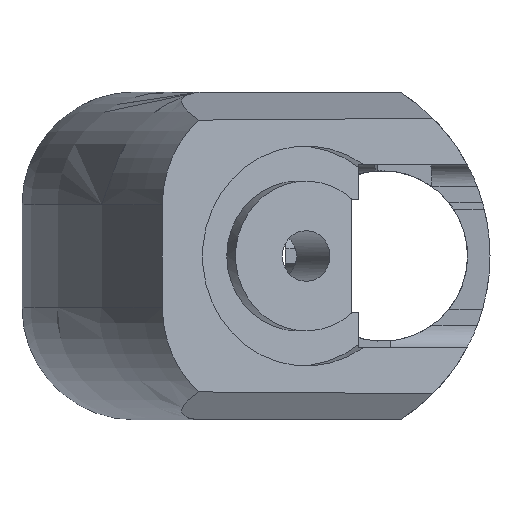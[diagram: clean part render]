
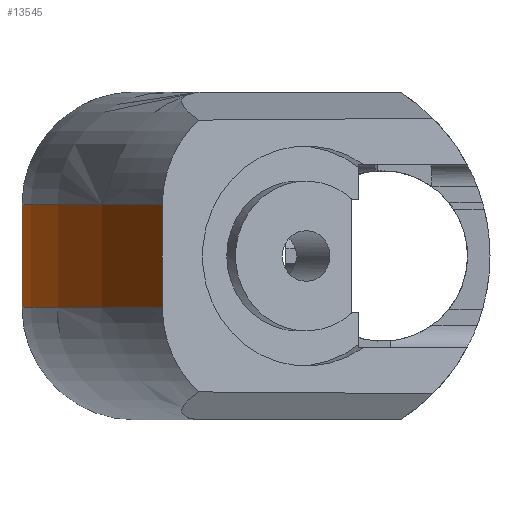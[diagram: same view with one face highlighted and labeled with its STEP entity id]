
A CAD part, left-side view. The second image highlights one B-rep face of the part: STEP entity #13545.
In plain terms, the highlighted cylindrical face has radius 197.297 mm (diameter 394.594 mm), a partial arc.
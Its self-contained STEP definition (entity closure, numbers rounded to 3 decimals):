
#157 = PLANE('',#158);
#158 = AXIS2_PLACEMENT_3D('',#159,#160,#161);
#159 = CARTESIAN_POINT('',(0.,63.5,-22.225));
#160 = DIRECTION('',(0.,-1.,0.));
#161 = DIRECTION('',(-1.,0.,0.));
#2285 = PLANE('',#2286);
#2286 = AXIS2_PLACEMENT_3D('',#2287,#2288,#2289);
#2287 = CARTESIAN_POINT('',(-209.55,44.45,-22.225));
#2288 = DIRECTION('',(0.943,0.334,0.)
  );
#2289 = DIRECTION('',(0.334,-0.943,0.)
  );
#2979 = TOROIDAL_SURFACE('',#2980,182.057,15.24);
#2980 = AXIS2_PLACEMENT_3D('',#2981,#2982,#2983);
#2981 = CARTESIAN_POINT('',(-124.968,-133.797,6.985));
#2982 = DIRECTION('',(0.,0.,-1.));
#2983 = DIRECTION('',(0.,1.,0.));
#4018 = VERTEX_POINT('',#4019);
#4019 = CARTESIAN_POINT('',(-124.968,63.5,6.985));
#4344 = EDGE_CURVE('',#4345,#4018,#4347,.T.);
#4345 = VERTEX_POINT('',#4346);
#4346 = CARTESIAN_POINT('',(-124.968,63.5,-6.985));
#4347 = SURFACE_CURVE('',#4348,(#4352,#4359),.PCURVE_S1.);
#4348 = LINE('',#4349,#4350);
#4349 = CARTESIAN_POINT('',(-124.968,63.5,-22.225));
#4350 = VECTOR('',#4351,1.);
#4351 = DIRECTION('',(0.,0.,1.));
#4352 = PCURVE('',#157,#4353);
#4353 = DEFINITIONAL_REPRESENTATION('',(#4354),#4358);
#4354 = LINE('',#4355,#4356);
#4355 = CARTESIAN_POINT('',(124.968,0.));
#4356 = VECTOR('',#4357,1.);
#4357 = DIRECTION('',(0.,-1.));
#4358 = ( GEOMETRIC_REPRESENTATION_CONTEXT(2) 
PARAMETRIC_REPRESENTATION_CONTEXT() REPRESENTATION_CONTEXT('2D SPACE',''
  ) );
#4359 = PCURVE('',#4360,#4365);
#4360 = CYLINDRICAL_SURFACE('',#4361,197.297);
#4361 = AXIS2_PLACEMENT_3D('',#4362,#4363,#4364);
#4362 = CARTESIAN_POINT('',(-124.968,-133.797,-22.225));
#4363 = DIRECTION('',(0.,0.,-1.));
#4364 = DIRECTION('',(1.,0.,0.));
#4365 = DEFINITIONAL_REPRESENTATION('',(#4366),#4370);
#4366 = LINE('',#4367,#4368);
#4367 = CARTESIAN_POINT('',(-1.571,0.));
#4368 = VECTOR('',#4369,1.);
#4369 = DIRECTION('',(-0.,-1.));
#4370 = ( GEOMETRIC_REPRESENTATION_CONTEXT(2) 
PARAMETRIC_REPRESENTATION_CONTEXT() REPRESENTATION_CONTEXT('2D SPACE',''
  ) );
#4468 = TOROIDAL_SURFACE('',#4469,182.057,15.24);
#4469 = AXIS2_PLACEMENT_3D('',#4470,#4471,#4472);
#4470 = CARTESIAN_POINT('',(-124.968,-133.797,-6.985));
#4471 = DIRECTION('',(0.,0.,1.));
#4472 = DIRECTION('',(0.,1.,0.));
#10113 = VERTEX_POINT('',#10114);
#10114 = CARTESIAN_POINT('',(-209.55,44.45,-6.985));
#10204 = EDGE_CURVE('',#10113,#10205,#10207,.T.);
#10205 = VERTEX_POINT('',#10206);
#10206 = CARTESIAN_POINT('',(-209.55,44.45,6.985));
#10207 = SURFACE_CURVE('',#10208,(#10212,#10219),.PCURVE_S1.);
#10208 = LINE('',#10209,#10210);
#10209 = CARTESIAN_POINT('',(-209.55,44.45,-22.225));
#10210 = VECTOR('',#10211,1.);
#10211 = DIRECTION('',(0.,0.,1.));
#10212 = PCURVE('',#2285,#10213);
#10213 = DEFINITIONAL_REPRESENTATION('',(#10214),#10218);
#10214 = LINE('',#10215,#10216);
#10215 = CARTESIAN_POINT('',(0.,-0.));
#10216 = VECTOR('',#10217,1.);
#10217 = DIRECTION('',(0.,-1.));
#10218 = ( GEOMETRIC_REPRESENTATION_CONTEXT(2) 
PARAMETRIC_REPRESENTATION_CONTEXT() REPRESENTATION_CONTEXT('2D SPACE',''
  ) );
#10219 = PCURVE('',#4360,#10220);
#10220 = DEFINITIONAL_REPRESENTATION('',(#10221),#10225);
#10221 = LINE('',#10222,#10223);
#10222 = CARTESIAN_POINT('',(-2.014,0.));
#10223 = VECTOR('',#10224,1.);
#10224 = DIRECTION('',(-0.,-1.));
#10225 = ( GEOMETRIC_REPRESENTATION_CONTEXT(2) 
PARAMETRIC_REPRESENTATION_CONTEXT() REPRESENTATION_CONTEXT('2D SPACE',''
  ) );
#11246 = EDGE_CURVE('',#4018,#10205,#11247,.T.);
#11247 = SURFACE_CURVE('',#11248,(#11253,#11260),.PCURVE_S1.);
#11248 = CIRCLE('',#11249,197.297);
#11249 = AXIS2_PLACEMENT_3D('',#11250,#11251,#11252);
#11250 = CARTESIAN_POINT('',(-124.968,-133.797,6.985));
#11251 = DIRECTION('',(0.,0.,1.));
#11252 = DIRECTION('',(0.,1.,0.));
#11253 = PCURVE('',#2979,#11254);
#11254 = DEFINITIONAL_REPRESENTATION('',(#11255),#11259);
#11255 = LINE('',#11256,#11257);
#11256 = CARTESIAN_POINT('',(-0.,6.283));
#11257 = VECTOR('',#11258,1.);
#11258 = DIRECTION('',(-1.,0.));
#11259 = ( GEOMETRIC_REPRESENTATION_CONTEXT(2) 
PARAMETRIC_REPRESENTATION_CONTEXT() REPRESENTATION_CONTEXT('2D SPACE',''
  ) );
#11260 = PCURVE('',#4360,#11261);
#11261 = DEFINITIONAL_REPRESENTATION('',(#11262),#11266);
#11262 = LINE('',#11263,#11264);
#11263 = CARTESIAN_POINT('',(-1.571,-29.21));
#11264 = VECTOR('',#11265,1.);
#11265 = DIRECTION('',(-1.,0.));
#11266 = ( GEOMETRIC_REPRESENTATION_CONTEXT(2) 
PARAMETRIC_REPRESENTATION_CONTEXT() REPRESENTATION_CONTEXT('2D SPACE',''
  ) );
#13545 = ADVANCED_FACE('',(#13546),#4360,.T.);
#13546 = FACE_BOUND('',#13547,.F.);
#13547 = EDGE_LOOP('',(#13548,#13549,#13550,#13551));
#13548 = ORIENTED_EDGE('',*,*,#4344,.T.);
#13549 = ORIENTED_EDGE('',*,*,#11246,.T.);
#13550 = ORIENTED_EDGE('',*,*,#10204,.F.);
#13551 = ORIENTED_EDGE('',*,*,#13552,.F.);
#13552 = EDGE_CURVE('',#4345,#10113,#13553,.T.);
#13553 = SURFACE_CURVE('',#13554,(#13559,#13566),.PCURVE_S1.);
#13554 = CIRCLE('',#13555,197.297);
#13555 = AXIS2_PLACEMENT_3D('',#13556,#13557,#13558);
#13556 = CARTESIAN_POINT('',(-124.968,-133.797,-6.985));
#13557 = DIRECTION('',(0.,0.,1.));
#13558 = DIRECTION('',(0.,1.,0.));
#13559 = PCURVE('',#4360,#13560);
#13560 = DEFINITIONAL_REPRESENTATION('',(#13561),#13565);
#13561 = LINE('',#13562,#13563);
#13562 = CARTESIAN_POINT('',(-1.571,-15.24));
#13563 = VECTOR('',#13564,1.);
#13564 = DIRECTION('',(-1.,0.));
#13565 = ( GEOMETRIC_REPRESENTATION_CONTEXT(2) 
PARAMETRIC_REPRESENTATION_CONTEXT() REPRESENTATION_CONTEXT('2D SPACE',''
  ) );
#13566 = PCURVE('',#4468,#13567);
#13567 = DEFINITIONAL_REPRESENTATION('',(#13568),#13572);
#13568 = LINE('',#13569,#13570);
#13569 = CARTESIAN_POINT('',(0.,6.283));
#13570 = VECTOR('',#13571,1.);
#13571 = DIRECTION('',(1.,0.));
#13572 = ( GEOMETRIC_REPRESENTATION_CONTEXT(2) 
PARAMETRIC_REPRESENTATION_CONTEXT() REPRESENTATION_CONTEXT('2D SPACE',''
  ) );
